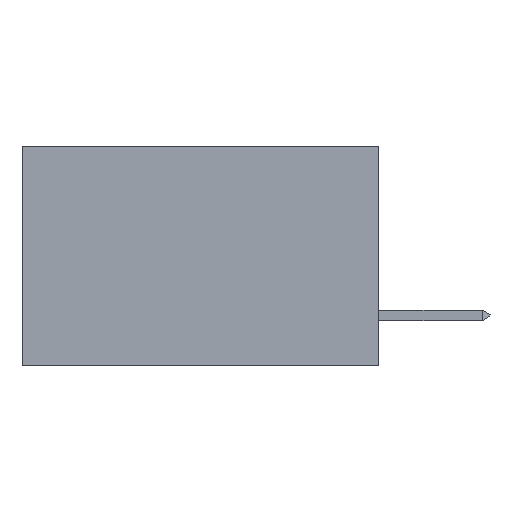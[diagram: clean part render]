
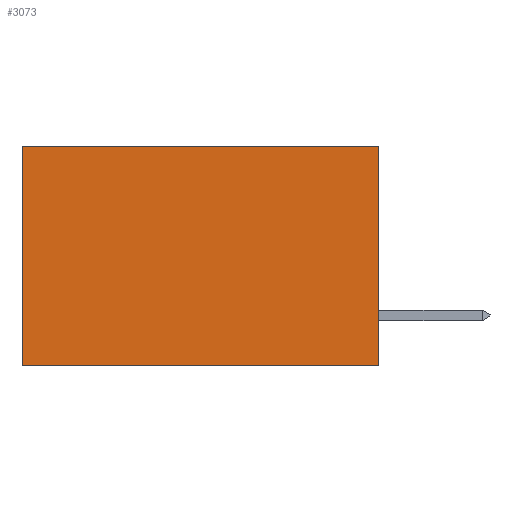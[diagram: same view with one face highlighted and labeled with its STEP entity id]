
A CAD part, left-side view. The second image highlights one B-rep face of the part: STEP entity #3073.
In plain terms, the highlighted planar face has unit normal (-1, 0, 0).
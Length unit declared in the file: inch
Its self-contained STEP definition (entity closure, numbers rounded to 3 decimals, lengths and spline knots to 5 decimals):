
#834 = CARTESIAN_POINT ( 'NONE',  ( 0.298, 0.6, -0.37 ) ) ;
#1379 = LINE ( 'NONE', #4313, #2672 ) ;
#2385 = VERTEX_POINT ( 'NONE', #5957 ) ;
#2672 = VECTOR ( 'NONE', #11500, 39.37008 ) ;
#3073 = ADVANCED_FACE ( 'NONE', ( #10997 ), #5396, .F. ) ;
#3296 = DIRECTION ( 'NONE',  ( 0., 1., 0. ) ) ;
#3414 = EDGE_CURVE ( 'NONE', #12232, #5953, #11798, .T. ) ;
#3554 = VECTOR ( 'NONE', #5754, 39.37008 ) ;
#3750 = AXIS2_PLACEMENT_3D ( 'NONE', #4461, #11656, #5487 ) ;
#4313 = CARTESIAN_POINT ( 'NONE',  ( 0.298, 0., 0. ) ) ;
#4461 = CARTESIAN_POINT ( 'NONE',  ( 0.298, 0., 0. ) ) ;
#4799 = ORIENTED_EDGE ( 'NONE', *, *, #8397, .T. ) ;
#5213 = EDGE_CURVE ( 'NONE', #11277, #12232, #1379, .T. ) ;
#5396 = PLANE ( 'NONE',  #3750 ) ;
#5439 = CARTESIAN_POINT ( 'NONE',  ( 0.298, 0.6, 0. ) ) ;
#5487 = DIRECTION ( 'NONE',  ( 0., 0., -1. ) ) ;
#5754 = DIRECTION ( 'NONE',  ( 0., 0., -1. ) ) ;
#5953 = VERTEX_POINT ( 'NONE', #834 ) ;
#5957 = CARTESIAN_POINT ( 'NONE',  ( 0.298, 0.6, 0. ) ) ;
#6091 = DIRECTION ( 'NONE',  ( 0., 1., 0. ) ) ;
#6606 = VECTOR ( 'NONE', #6091, 39.37008 ) ;
#7163 = CARTESIAN_POINT ( 'NONE',  ( 0.298, 0., 0. ) ) ;
#7985 = CARTESIAN_POINT ( 'NONE',  ( 0.298, 0., 0. ) ) ;
#8397 = EDGE_CURVE ( 'NONE', #2385, #5953, #11237, .T. ) ;
#8534 = CARTESIAN_POINT ( 'NONE',  ( 0.298, 0., -0.37 ) ) ;
#10018 = CARTESIAN_POINT ( 'NONE',  ( 0.298, 0., -0.37 ) ) ;
#10343 = VECTOR ( 'NONE', #3296, 39.37008 ) ;
#10846 = EDGE_LOOP ( 'NONE', ( #4799, #11407, #12491, #12351 ) ) ;
#10997 = FACE_OUTER_BOUND ( 'NONE', #10846, .T. ) ;
#11237 = LINE ( 'NONE', #5439, #3554 ) ;
#11277 = VERTEX_POINT ( 'NONE', #7985 ) ;
#11407 = ORIENTED_EDGE ( 'NONE', *, *, #3414, .F. ) ;
#11500 = DIRECTION ( 'NONE',  ( 0., 0., -1. ) ) ;
#11656 = DIRECTION ( 'NONE',  ( 1., 0., 0. ) ) ;
#11798 = LINE ( 'NONE', #8534, #10343 ) ;
#11932 = LINE ( 'NONE', #7163, #6606 ) ;
#12232 = VERTEX_POINT ( 'NONE', #10018 ) ;
#12351 = ORIENTED_EDGE ( 'NONE', *, *, #13015, .T. ) ;
#12491 = ORIENTED_EDGE ( 'NONE', *, *, #5213, .F. ) ;
#13015 = EDGE_CURVE ( 'NONE', #11277, #2385, #11932, .T. ) ;
